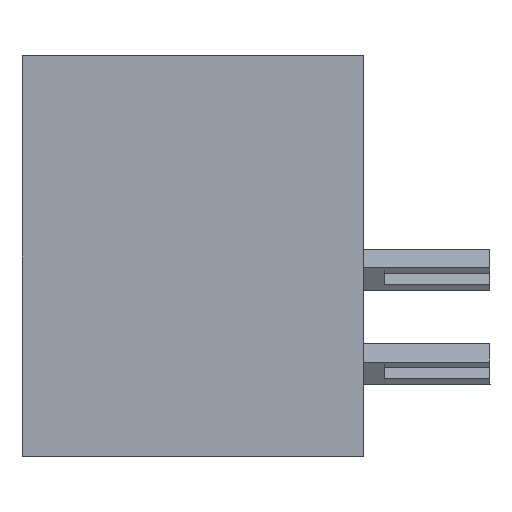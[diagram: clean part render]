
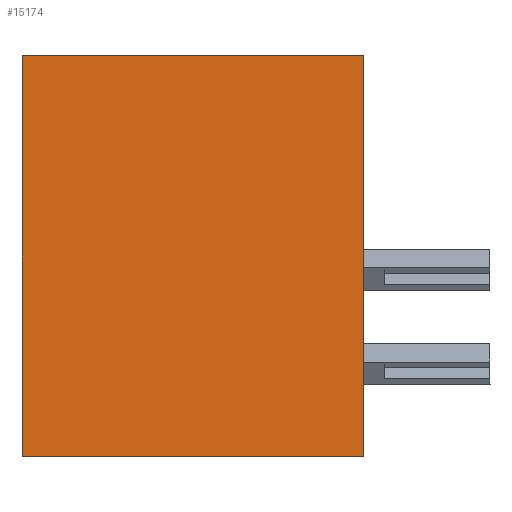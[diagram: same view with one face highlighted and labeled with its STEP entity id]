
A CAD part, left-side view. The second image highlights one B-rep face of the part: STEP entity #15174.
In plain terms, the highlighted planar face has unit normal (-1, 0, 0).
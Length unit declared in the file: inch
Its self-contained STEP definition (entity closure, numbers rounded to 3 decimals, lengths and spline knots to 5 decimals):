
#666 = ORIENTED_EDGE ( 'NONE', *, *, #1666, .T. ) ;
#827 = EDGE_LOOP ( 'NONE', ( #13170, #17917, #19662, #666 ) ) ;
#1338 = CARTESIAN_POINT ( 'NONE',  ( 0., 0.453, -0.531 ) ) ;
#1666 = EDGE_CURVE ( 'NONE', #24639, #19448, #14719, .T. ) ;
#2717 = VECTOR ( 'NONE', #8495, 39.37008 ) ;
#3630 = CARTESIAN_POINT ( 'NONE',  ( 0., 0.453, 0. ) ) ;
#4219 = AXIS2_PLACEMENT_3D ( 'NONE', #3630, #26858, #13779 ) ;
#5036 = LINE ( 'NONE', #11880, #23208 ) ;
#5907 = DIRECTION ( 'NONE',  ( 0., 0., 1. ) ) ;
#8204 = FACE_OUTER_BOUND ( 'NONE', #827, .T. ) ;
#8264 = VERTEX_POINT ( 'NONE', #23218 ) ;
#8495 = DIRECTION ( 'NONE',  ( 0., -1., 0. ) ) ;
#9741 = VECTOR ( 'NONE', #17398, 39.37008 ) ;
#10902 = CARTESIAN_POINT ( 'NONE',  ( 0., 0.453, 0. ) ) ;
#11880 = CARTESIAN_POINT ( 'NONE',  ( 0., 0., 0. ) ) ;
#12220 = EDGE_CURVE ( 'NONE', #24639, #25356, #15060, .T. ) ;
#13170 = ORIENTED_EDGE ( 'NONE', *, *, #20205, .T. ) ;
#13304 = CARTESIAN_POINT ( 'NONE',  ( 0., 0.453, 0. ) ) ;
#13779 = DIRECTION ( 'NONE',  ( 0., 0., -1. ) ) ;
#14096 = DIRECTION ( 'NONE',  ( 0., -1., 0. ) ) ;
#14719 = LINE ( 'NONE', #1338, #15041 ) ;
#15041 = VECTOR ( 'NONE', #14096, 39.37008 ) ;
#15060 = LINE ( 'NONE', #13304, #9741 ) ;
#15174 = ADVANCED_FACE ( 'NONE', ( #8204 ), #24519, .F. ) ;
#15886 = CARTESIAN_POINT ( 'NONE',  ( 0., 0.453, -0.531 ) ) ;
#17398 = DIRECTION ( 'NONE',  ( 0., 0., 1. ) ) ;
#17917 = ORIENTED_EDGE ( 'NONE', *, *, #19782, .F. ) ;
#19448 = VERTEX_POINT ( 'NONE', #26387 ) ;
#19662 = ORIENTED_EDGE ( 'NONE', *, *, #12220, .F. ) ;
#19782 = EDGE_CURVE ( 'NONE', #25356, #8264, #23556, .T. ) ;
#20205 = EDGE_CURVE ( 'NONE', #19448, #8264, #5036, .T. ) ;
#21182 = CARTESIAN_POINT ( 'NONE',  ( 0., 0.453, 0. ) ) ;
#23208 = VECTOR ( 'NONE', #5907, 39.37008 ) ;
#23218 = CARTESIAN_POINT ( 'NONE',  ( 0., 0., 0. ) ) ;
#23556 = LINE ( 'NONE', #21182, #2717 ) ;
#24519 = PLANE ( 'NONE',  #4219 ) ;
#24639 = VERTEX_POINT ( 'NONE', #15886 ) ;
#25356 = VERTEX_POINT ( 'NONE', #10902 ) ;
#26387 = CARTESIAN_POINT ( 'NONE',  ( 0., 0., -0.531 ) ) ;
#26858 = DIRECTION ( 'NONE',  ( 1., 0., 0. ) ) ;
